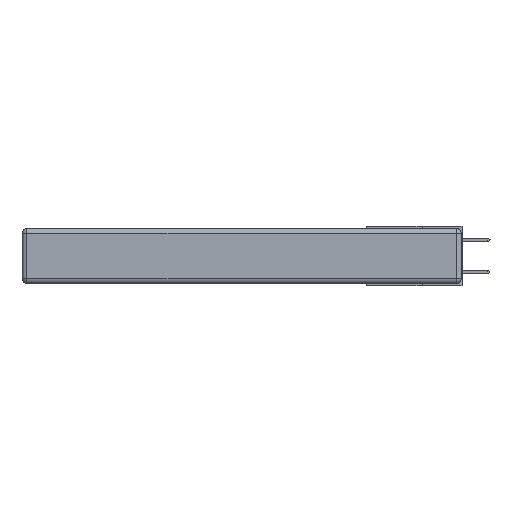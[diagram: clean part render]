
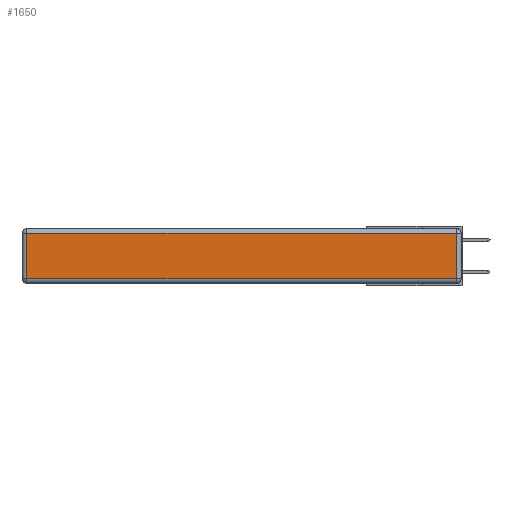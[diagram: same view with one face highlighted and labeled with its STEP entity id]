
A CAD part, left-side view. The second image highlights one B-rep face of the part: STEP entity #1650.
In plain terms, the highlighted planar face has unit normal (-1, 0, 0).
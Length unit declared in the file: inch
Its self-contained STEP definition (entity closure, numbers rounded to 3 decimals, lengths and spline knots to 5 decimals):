
#582 = VERTEX_POINT ( 'NONE', #16031 ) ;
#1475 = ORIENTED_EDGE ( 'NONE', *, *, #4132, .T. ) ;
#1650 = ADVANCED_FACE ( 'NONE', ( #7858 ), #3064, .T. ) ;
#1745 = VERTEX_POINT ( 'NONE', #14513 ) ;
#1792 = DIRECTION ( 'NONE',  ( 0., 1., 0. ) ) ;
#2936 = EDGE_LOOP ( 'NONE', ( #7648, #1475, #4944, #10144 ) ) ;
#3064 = PLANE ( 'NONE',  #6761 ) ;
#3450 = VERTEX_POINT ( 'NONE', #8969 ) ;
#3937 = VECTOR ( 'NONE', #7375, 39.37008 ) ;
#4132 = EDGE_CURVE ( 'NONE', #10215, #3450, #9899, .T. ) ;
#4299 = DIRECTION ( 'NONE',  ( 0., 0., 1. ) ) ;
#4451 = CARTESIAN_POINT ( 'NONE',  ( 0., 0., -0.343 ) ) ;
#4944 = ORIENTED_EDGE ( 'NONE', *, *, #6180, .T. ) ;
#5530 = DIRECTION ( 'NONE',  ( 0., 0., 1. ) ) ;
#5961 = LINE ( 'NONE', #15474, #12004 ) ;
#6074 = LINE ( 'NONE', #7473, #3937 ) ;
#6180 = EDGE_CURVE ( 'NONE', #3450, #582, #5961, .T. ) ;
#6761 = AXIS2_PLACEMENT_3D ( 'NONE', #4451, #14328, #5530 ) ;
#6807 = CARTESIAN_POINT ( 'NONE',  ( 0., 0.03, -0.313 ) ) ;
#7331 = EDGE_CURVE ( 'NONE', #1745, #10215, #6074, .T. ) ;
#7375 = DIRECTION ( 'NONE',  ( 0., -1., 0. ) ) ;
#7473 = CARTESIAN_POINT ( 'NONE',  ( 0., 0., -0.313 ) ) ;
#7648 = ORIENTED_EDGE ( 'NONE', *, *, #7331, .T. ) ;
#7858 = FACE_OUTER_BOUND ( 'NONE', #2936, .T. ) ;
#8003 = EDGE_CURVE ( 'NONE', #582, #1745, #11980, .T. ) ;
#8105 = DIRECTION ( 'NONE',  ( 0., 0., -1. ) ) ;
#8969 = CARTESIAN_POINT ( 'NONE',  ( 0., 0.03, -0.03 ) ) ;
#9899 = LINE ( 'NONE', #12744, #12421 ) ;
#10144 = ORIENTED_EDGE ( 'NONE', *, *, #8003, .T. ) ;
#10215 = VERTEX_POINT ( 'NONE', #6807 ) ;
#10804 = CARTESIAN_POINT ( 'NONE',  ( 0., 2.72, -0.343 ) ) ;
#11980 = LINE ( 'NONE', #10804, #13856 ) ;
#12004 = VECTOR ( 'NONE', #1792, 39.37008 ) ;
#12421 = VECTOR ( 'NONE', #4299, 39.37008 ) ;
#12744 = CARTESIAN_POINT ( 'NONE',  ( 0., 0.03, -0.343 ) ) ;
#13856 = VECTOR ( 'NONE', #8105, 39.37008 ) ;
#14328 = DIRECTION ( 'NONE',  ( -1., 0., 0. ) ) ;
#14513 = CARTESIAN_POINT ( 'NONE',  ( 0., 2.72, -0.313 ) ) ;
#15474 = CARTESIAN_POINT ( 'NONE',  ( 0., 2.75, -0.03 ) ) ;
#16031 = CARTESIAN_POINT ( 'NONE',  ( 0., 2.72, -0.03 ) ) ;
